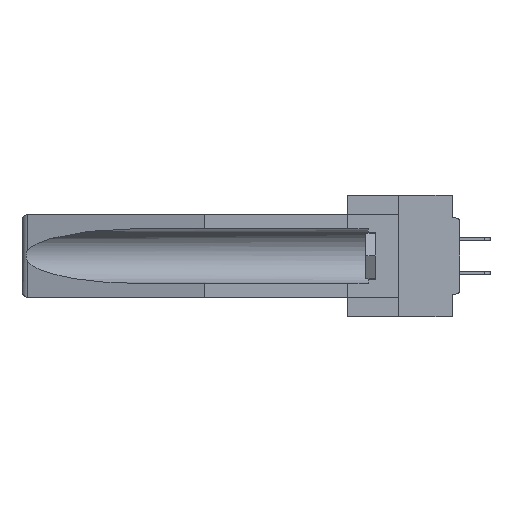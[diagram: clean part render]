
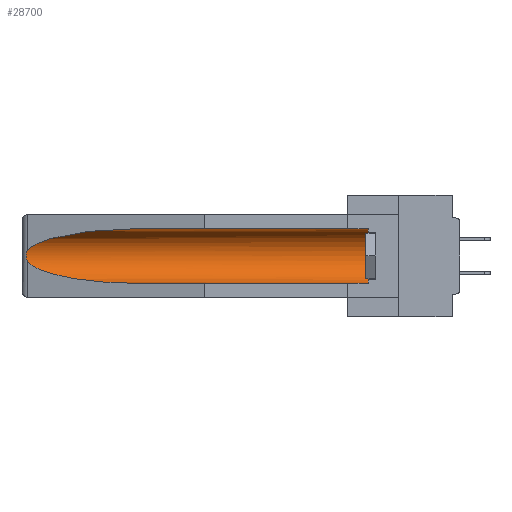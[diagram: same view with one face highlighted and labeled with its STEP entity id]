
A CAD part, left-side view. The second image highlights one B-rep face of the part: STEP entity #28700.
In plain terms, the highlighted cylindrical face has radius 2.857 mm (diameter 5.715 mm), a partial arc.
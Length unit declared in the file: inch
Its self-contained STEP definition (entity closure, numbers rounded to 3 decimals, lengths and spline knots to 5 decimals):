
#1190 = CARTESIAN_POINT ( 'NONE',  ( 0.21114, 1.30732, -0.059 ) ) ;
#1646 = DIRECTION ( 'NONE',  ( 0., 1., 0. ) ) ;
#1828 = AXIS2_PLACEMENT_3D ( 'NONE', #27107, #18118, #29827 ) ;
#3280 = CARTESIAN_POINT ( 'NONE',  ( 0.2673, 1.5327, -0.16383 ) ) ;
#3502 = EDGE_CURVE ( 'NONE', #5981, #8273, #35676, .T. ) ;
#4202 = CARTESIAN_POINT ( 'NONE',  ( 0.155, 0.126, -0.059 ) ) ;
#4816 = CARTESIAN_POINT ( 'NONE',  ( 0.26537, 1.52718, -0.19328 ) ) ;
#5981 = VERTEX_POINT ( 'NONE', #28112 ) ;
#6215 = CARTESIAN_POINT ( 'NONE',  ( 0.26597, 1.5296, -0.19026 ) ) ;
#6826 = EDGE_CURVE ( 'NONE', #8273, #25876, #32829, .T. ) ;
#6951 = CARTESIAN_POINT ( 'NONE',  ( 0.155, 1.07973, -0.059 ) ) ;
#7189 = CARTESIAN_POINT ( 'NONE',  ( 0.155, 1.07973, -0.284 ) ) ;
#7721 = DIRECTION ( 'NONE',  ( 0., 1., 0. ) ) ;
#8273 = VERTEX_POINT ( 'NONE', #12475 ) ;
#8303 = ORIENTED_EDGE ( 'NONE', *, *, #10660, .F. ) ;
#8797 = CARTESIAN_POINT ( 'NONE',  ( 0.2675, 1.53308, -0.17534 ) ) ;
#10660 = EDGE_CURVE ( 'NONE', #35661, #33441, #14585, .T. ) ;
#11795 = ORIENTED_EDGE ( 'NONE', *, *, #6826, .T. ) ;
#11914 = CARTESIAN_POINT ( 'NONE',  ( 0.26537, 1.52718, -0.19328 ) ) ;
#12307 = CARTESIAN_POINT ( 'NONE',  ( 0.26597, 1.52961, -0.15275 ) ) ;
#12475 = CARTESIAN_POINT ( 'NONE',  ( 0.26537, 1.52718, -0.14972 ) ) ;
#13553 = CARTESIAN_POINT ( 'NONE',  ( 0.26537, 1.52718, -0.19328 ) ) ;
#13625 = FACE_OUTER_BOUND ( 'NONE', #29071, .T. ) ;
#14585 = LINE ( 'NONE', #20201, #33050 ) ;
#15162 = CARTESIAN_POINT ( 'NONE',  ( 0.26654, 1.53092, -0.15636 ) ) ;
#15517 = CARTESIAN_POINT ( 'NONE',  ( 0.25451, 1.48313, -0.09465 ) ) ;
#16840 = CARTESIAN_POINT ( 'NONE',  ( 0.25451, 1.48313, -0.24835 ) ) ;
#17595 = DIRECTION ( 'NONE',  ( 0., 0., 1. ) ) ;
#18118 = DIRECTION ( 'NONE',  ( 0., -1., 0. ) ) ;
#18160 = CARTESIAN_POINT ( 'NONE',  ( 0.26655, 1.53094, -0.18657 ) ) ;
#18785 = CARTESIAN_POINT ( 'NONE',  ( 0.155, -0.30754, -0.059 ) ) ;
#19209 = CARTESIAN_POINT ( 'NONE',  ( 0.155, -0.30754, -0.1715 ) ) ;
#20201 = CARTESIAN_POINT ( 'NONE',  ( 0.155, -0.30754, -0.284 ) ) ;
#20503 = ORIENTED_EDGE ( 'NONE', *, *, #3502, .T. ) ;
#22954 = VERTEX_POINT ( 'NONE', #4202 ) ;
#23932 = CARTESIAN_POINT ( 'NONE',  ( 0.2673, 1.53269, -0.17917 ) ) ;
#24534 = LINE ( 'NONE', #18785, #35136 ) ;
#25832 = CARTESIAN_POINT ( 'NONE',  ( 0.155, 1.07973, -0.284 ) ) ;
#25876 = VERTEX_POINT ( 'NONE', #13553 ) ;
#26542 = CYLINDRICAL_SURFACE ( 'NONE', #36344, 0.1125 ) ;
#27107 = CARTESIAN_POINT ( 'NONE',  ( 0.155, 0.126, -0.1715 ) ) ;
#28112 = CARTESIAN_POINT ( 'NONE',  ( 0.155, 1.07973, -0.059 ) ) ;
#28700 = ADVANCED_FACE ( 'NONE', ( #13625 ), #26542, .F. ) ;
#29071 = EDGE_LOOP ( 'NONE', ( #20503, #11795, #36141, #8303, #34111, #34554 ) ) ;
#29111 = CARTESIAN_POINT ( 'NONE',  ( 0.155, 0.126, -0.284 ) ) ;
#29827 = DIRECTION ( 'NONE',  ( 0., 0., 1. ) ) ;
#29836 = DIRECTION ( 'NONE',  ( 0., 1., 0. ) ) ;
#32784 = EDGE_CURVE ( 'NONE', #35661, #22954, #36329, .T. ) ;
#32829 = B_SPLINE_CURVE_WITH_KNOTS ( 'NONE', 3,
 ( #35915, #12307, #15162, #3280, #35791, #8797, #23932, #18160, #6215, #11914 ),
 .UNSPECIFIED., .F., .F.,
 ( 4, 2, 2, 2, 4 ),
 ( 0., 0.00029, 0.00058, 0.00087, 0.00117 ),
 .UNSPECIFIED. ) ;
#33050 = VECTOR ( 'NONE', #29836, 39.37008 ) ;
#33441 = VERTEX_POINT ( 'NONE', #7189 ) ;
#34111 = ORIENTED_EDGE ( 'NONE', *, *, #32784, .T. ) ;
#34554 = ORIENTED_EDGE ( 'NONE', *, *, #36867, .T. ) ;
#34753 =( BOUNDED_CURVE ( )  B_SPLINE_CURVE ( 3, ( #4816, #16840, #37416, #25832 ),
 .UNSPECIFIED., .F., .F. ) 
 B_SPLINE_CURVE_WITH_KNOTS ( ( 4, 4 ),
 ( 0.1948, 1.5708 ),
 .UNSPECIFIED. ) 
 CURVE ( )  GEOMETRIC_REPRESENTATION_ITEM ( )  RATIONAL_B_SPLINE_CURVE ( ( 1., 0.848, 0.848, 1. ) ) 
 REPRESENTATION_ITEM ( '' )  );
#35136 = VECTOR ( 'NONE', #7721, 39.37008 ) ;
#35204 = EDGE_CURVE ( 'NONE', #25876, #33441, #34753, .T. ) ;
#35661 = VERTEX_POINT ( 'NONE', #29111 ) ;
#35676 =( BOUNDED_CURVE ( )  B_SPLINE_CURVE ( 3, ( #6951, #1190, #15517, #36130 ),
 .UNSPECIFIED., .F., .F. ) 
 B_SPLINE_CURVE_WITH_KNOTS ( ( 4, 4 ),
 ( 4.71239, 6.08839 ),
 .UNSPECIFIED. ) 
 CURVE ( )  GEOMETRIC_REPRESENTATION_ITEM ( )  RATIONAL_B_SPLINE_CURVE ( ( 1., 0.848, 0.848, 1. ) ) 
 REPRESENTATION_ITEM ( '' )  );
#35791 = CARTESIAN_POINT ( 'NONE',  ( 0.2675, 1.53308, -0.16763 ) ) ;
#35915 = CARTESIAN_POINT ( 'NONE',  ( 0.26537, 1.52718, -0.14972 ) ) ;
#36130 = CARTESIAN_POINT ( 'NONE',  ( 0.26537, 1.52718, -0.14972 ) ) ;
#36141 = ORIENTED_EDGE ( 'NONE', *, *, #35204, .T. ) ;
#36329 = CIRCLE ( 'NONE', #1828, 0.1125 ) ;
#36344 = AXIS2_PLACEMENT_3D ( 'NONE', #19209, #1646, #17595 ) ;
#36867 = EDGE_CURVE ( 'NONE', #22954, #5981, #24534, .T. ) ;
#37416 = CARTESIAN_POINT ( 'NONE',  ( 0.21114, 1.30732, -0.284 ) ) ;
